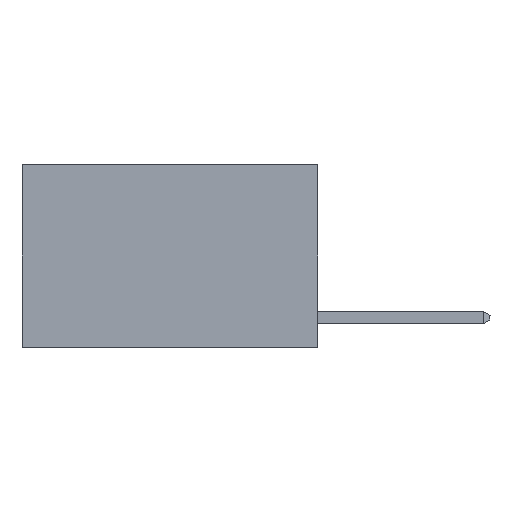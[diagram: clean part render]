
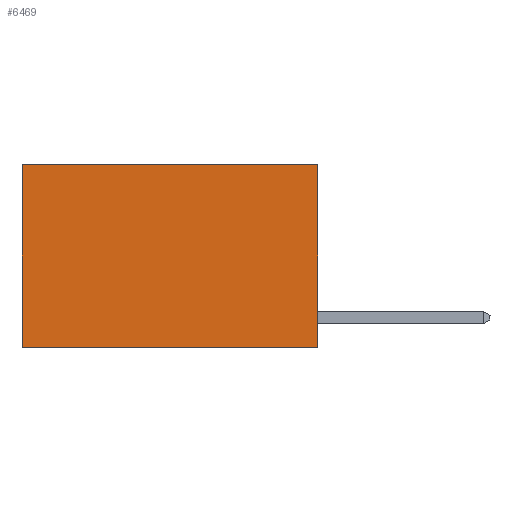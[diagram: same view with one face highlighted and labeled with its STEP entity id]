
A CAD part, left-side view. The second image highlights one B-rep face of the part: STEP entity #6469.
In plain terms, the highlighted planar face has unit normal (-1, 0, 0).
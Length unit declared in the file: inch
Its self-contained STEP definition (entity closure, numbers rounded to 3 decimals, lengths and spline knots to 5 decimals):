
#1036 = EDGE_CURVE ( 'NONE', #9586, #8113, #4932, .T. ) ;
#1306 = CARTESIAN_POINT ( 'NONE',  ( 0.2625, 0.6, -0.37 ) ) ;
#1514 = EDGE_CURVE ( 'NONE', #4033, #8113, #11465, .T. ) ;
#1756 = CARTESIAN_POINT ( 'NONE',  ( 0.2625, 0., -0.37 ) ) ;
#1883 = VECTOR ( 'NONE', #5987, 39.37008 ) ;
#2285 = VERTEX_POINT ( 'NONE', #8012 ) ;
#2869 = CARTESIAN_POINT ( 'NONE',  ( 0.2625, 0.6, 0. ) ) ;
#3169 = LINE ( 'NONE', #11899, #1883 ) ;
#3430 = VECTOR ( 'NONE', #3904, 39.37008 ) ;
#3791 = CARTESIAN_POINT ( 'NONE',  ( 0.2625, 0.6, 0. ) ) ;
#3904 = DIRECTION ( 'NONE',  ( 0., 0., -1. ) ) ;
#4033 = VERTEX_POINT ( 'NONE', #1756 ) ;
#4505 = AXIS2_PLACEMENT_3D ( 'NONE', #12484, #5519, #10054 ) ;
#4533 = VECTOR ( 'NONE', #8843, 39.37008 ) ;
#4932 = LINE ( 'NONE', #2869, #3430 ) ;
#5519 = DIRECTION ( 'NONE',  ( 1., 0., 0. ) ) ;
#5560 = LINE ( 'NONE', #6564, #9877 ) ;
#5987 = DIRECTION ( 'NONE',  ( 0., 0., -1. ) ) ;
#6469 = ADVANCED_FACE ( 'NONE', ( #7732 ), #12436, .F. ) ;
#6547 = CARTESIAN_POINT ( 'NONE',  ( 0.2625, 0., -0.37 ) ) ;
#6564 = CARTESIAN_POINT ( 'NONE',  ( 0.2625, 0., 0. ) ) ;
#7051 = EDGE_CURVE ( 'NONE', #2285, #9586, #5560, .T. ) ;
#7732 = FACE_OUTER_BOUND ( 'NONE', #11637, .T. ) ;
#7917 = ORIENTED_EDGE ( 'NONE', *, *, #7051, .T. ) ;
#8012 = CARTESIAN_POINT ( 'NONE',  ( 0.2625, 0., 0. ) ) ;
#8113 = VERTEX_POINT ( 'NONE', #1306 ) ;
#8756 = DIRECTION ( 'NONE',  ( 0., 1., 0. ) ) ;
#8843 = DIRECTION ( 'NONE',  ( 0., 1., 0. ) ) ;
#9586 = VERTEX_POINT ( 'NONE', #3791 ) ;
#9877 = VECTOR ( 'NONE', #8756, 39.37008 ) ;
#10054 = DIRECTION ( 'NONE',  ( 0., 0., -1. ) ) ;
#11133 = ORIENTED_EDGE ( 'NONE', *, *, #11287, .F. ) ;
#11287 = EDGE_CURVE ( 'NONE', #2285, #4033, #3169, .T. ) ;
#11465 = LINE ( 'NONE', #6547, #4533 ) ;
#11637 = EDGE_LOOP ( 'NONE', ( #12879, #11924, #11133, #7917 ) ) ;
#11899 = CARTESIAN_POINT ( 'NONE',  ( 0.2625, 0., 0. ) ) ;
#11924 = ORIENTED_EDGE ( 'NONE', *, *, #1514, .F. ) ;
#12436 = PLANE ( 'NONE',  #4505 ) ;
#12484 = CARTESIAN_POINT ( 'NONE',  ( 0.2625, 0., 0. ) ) ;
#12879 = ORIENTED_EDGE ( 'NONE', *, *, #1036, .T. ) ;
